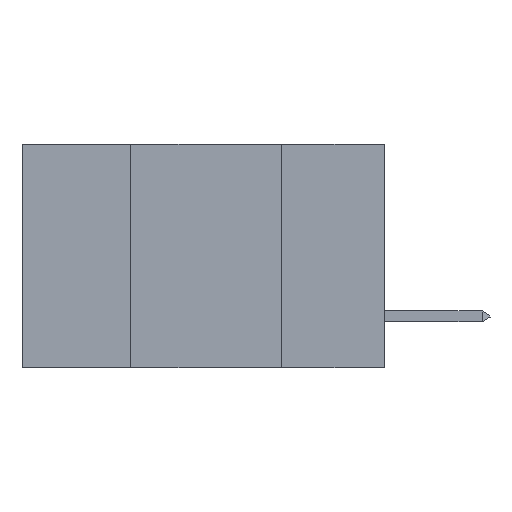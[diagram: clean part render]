
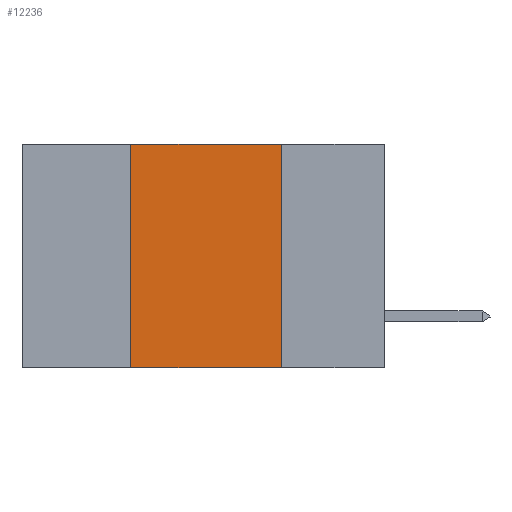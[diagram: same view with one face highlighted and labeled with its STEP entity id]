
A CAD part, left-side view. The second image highlights one B-rep face of the part: STEP entity #12236.
In plain terms, the highlighted planar face has unit normal (-1, 0, 0).
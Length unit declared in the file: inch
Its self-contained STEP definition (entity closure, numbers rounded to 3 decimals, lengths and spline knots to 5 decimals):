
#1363 = PLANE ( 'NONE',  #12047 ) ;
#1409 = VERTEX_POINT ( 'NONE', #14225 ) ;
#1861 = ORIENTED_EDGE ( 'NONE', *, *, #14179, .T. ) ;
#2490 = LINE ( 'NONE', #16091, #16029 ) ;
#3203 = CARTESIAN_POINT ( 'NONE',  ( 0., 0.6, 0. ) ) ;
#4535 = CARTESIAN_POINT ( 'NONE',  ( 0., 0.17, 0. ) ) ;
#4855 = VECTOR ( 'NONE', #16191, 39.37008 ) ;
#5160 = VERTEX_POINT ( 'NONE', #4535 ) ;
#5962 = VECTOR ( 'NONE', #23522, 39.37008 ) ;
#7228 = DIRECTION ( 'NONE',  ( 0., 0., -1. ) ) ;
#7399 = CARTESIAN_POINT ( 'NONE',  ( 0., 0.6, -0.37 ) ) ;
#8684 = DIRECTION ( 'NONE',  ( 0., 0., -1. ) ) ;
#9116 = DIRECTION ( 'NONE',  ( 1., 0., 0. ) ) ;
#9251 = EDGE_CURVE ( 'NONE', #14727, #18567, #9430, .T. ) ;
#9430 = LINE ( 'NONE', #17893, #5962 ) ;
#11866 = ORIENTED_EDGE ( 'NONE', *, *, #15680, .F. ) ;
#12047 = AXIS2_PLACEMENT_3D ( 'NONE', #3203, #9116, #7228 ) ;
#12236 = ADVANCED_FACE ( 'NONE', ( #14839 ), #1363, .F. ) ;
#12887 = EDGE_LOOP ( 'NONE', ( #17189, #11866, #19280, #1861 ) ) ;
#14179 = EDGE_CURVE ( 'NONE', #14727, #1409, #19345, .T. ) ;
#14225 = CARTESIAN_POINT ( 'NONE',  ( 0., 0.17, -0.37 ) ) ;
#14727 = VERTEX_POINT ( 'NONE', #17711 ) ;
#14839 = FACE_OUTER_BOUND ( 'NONE', #12887, .T. ) ;
#14995 = VECTOR ( 'NONE', #20839, 39.37008 ) ;
#15680 = EDGE_CURVE ( 'NONE', #18567, #5160, #18668, .T. ) ;
#16029 = VECTOR ( 'NONE', #8684, 39.37008 ) ;
#16091 = CARTESIAN_POINT ( 'NONE',  ( 0., 0.17, 0. ) ) ;
#16191 = DIRECTION ( 'NONE',  ( 0., -1., 0. ) ) ;
#17189 = ORIENTED_EDGE ( 'NONE', *, *, #23662, .F. ) ;
#17711 = CARTESIAN_POINT ( 'NONE',  ( 0., 0.42, -0.37 ) ) ;
#17893 = CARTESIAN_POINT ( 'NONE',  ( 0., 0.42, 0. ) ) ;
#18567 = VERTEX_POINT ( 'NONE', #19036 ) ;
#18668 = LINE ( 'NONE', #23416, #4855 ) ;
#19036 = CARTESIAN_POINT ( 'NONE',  ( 0., 0.42, 0. ) ) ;
#19280 = ORIENTED_EDGE ( 'NONE', *, *, #9251, .F. ) ;
#19345 = LINE ( 'NONE', #7399, #14995 ) ;
#20839 = DIRECTION ( 'NONE',  ( 0., -1., 0. ) ) ;
#23416 = CARTESIAN_POINT ( 'NONE',  ( 0., 0.6, 0. ) ) ;
#23522 = DIRECTION ( 'NONE',  ( 0., 0., 1. ) ) ;
#23662 = EDGE_CURVE ( 'NONE', #5160, #1409, #2490, .T. ) ;
